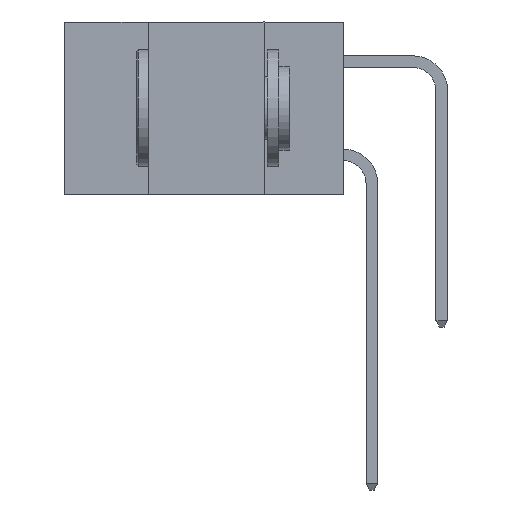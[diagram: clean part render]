
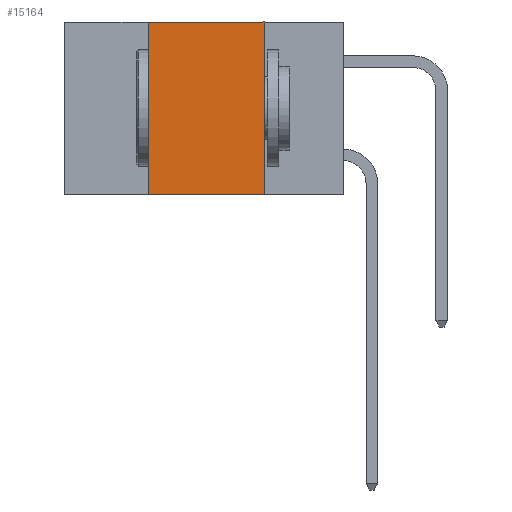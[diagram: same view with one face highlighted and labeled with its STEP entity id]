
A CAD part, left-side view. The second image highlights one B-rep face of the part: STEP entity #15164.
In plain terms, the highlighted planar face has unit normal (-1, 0, 0).
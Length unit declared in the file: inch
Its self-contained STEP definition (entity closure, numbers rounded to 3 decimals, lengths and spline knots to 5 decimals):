
#13 = DIRECTION ( 'NONE',  ( 0., 0., -1. ) ) ;
#141 = LINE ( 'NONE', #6042, #16493 ) ;
#431 = EDGE_CURVE ( 'NONE', #6835, #19722, #13069, .T. ) ;
#673 = ORIENTED_EDGE ( 'NONE', *, *, #8727, .F. ) ;
#1235 = CARTESIAN_POINT ( 'NONE',  ( 0., 0.42, -0.37 ) ) ;
#2145 = ORIENTED_EDGE ( 'NONE', *, *, #431, .T. ) ;
#2533 = EDGE_CURVE ( 'NONE', #6835, #9388, #14543, .T. ) ;
#3103 = PLANE ( 'NONE',  #10403 ) ;
#4089 = DIRECTION ( 'NONE',  ( 0., -1., 0. ) ) ;
#4337 = ORIENTED_EDGE ( 'NONE', *, *, #9751, .F. ) ;
#5850 = VERTEX_POINT ( 'NONE', #9584 ) ;
#5993 = VECTOR ( 'NONE', #4089, 39.37008 ) ;
#6042 = CARTESIAN_POINT ( 'NONE',  ( 0., 0.17, -0.37 ) ) ;
#6835 = VERTEX_POINT ( 'NONE', #10335 ) ;
#7136 = CARTESIAN_POINT ( 'NONE',  ( 0., 0.6, 0. ) ) ;
#7593 = DIRECTION ( 'NONE',  ( 0., 0., -1. ) ) ;
#7647 = CARTESIAN_POINT ( 'NONE',  ( 0., 0.6, -0.37 ) ) ;
#8727 = EDGE_CURVE ( 'NONE', #9388, #5850, #14105, .T. ) ;
#9280 = DIRECTION ( 'NONE',  ( 1., 0., 0. ) ) ;
#9388 = VERTEX_POINT ( 'NONE', #15934 ) ;
#9390 = ORIENTED_EDGE ( 'NONE', *, *, #2533, .F. ) ;
#9470 = CARTESIAN_POINT ( 'NONE',  ( 0., 0.17, -0.37 ) ) ;
#9584 = CARTESIAN_POINT ( 'NONE',  ( 0., 0.17, 0. ) ) ;
#9751 = EDGE_CURVE ( 'NONE', #5850, #19722, #141, .T. ) ;
#10335 = CARTESIAN_POINT ( 'NONE',  ( 0., 0.42, -0.37 ) ) ;
#10403 = AXIS2_PLACEMENT_3D ( 'NONE', #12274, #9280, #13 ) ;
#11241 = DIRECTION ( 'NONE',  ( 0., -1., 0. ) ) ;
#12026 = FACE_OUTER_BOUND ( 'NONE', #19530, .T. ) ;
#12274 = CARTESIAN_POINT ( 'NONE',  ( 0., 0.6, 0. ) ) ;
#12603 = VECTOR ( 'NONE', #11241, 39.37008 ) ;
#13069 = LINE ( 'NONE', #7647, #12603 ) ;
#14105 = LINE ( 'NONE', #7136, #5993 ) ;
#14543 = LINE ( 'NONE', #1235, #19088 ) ;
#15164 = ADVANCED_FACE ( 'NONE', ( #12026 ), #3103, .F. ) ;
#15934 = CARTESIAN_POINT ( 'NONE',  ( 0., 0.42, 0. ) ) ;
#16493 = VECTOR ( 'NONE', #7593, 39.37008 ) ;
#18035 = DIRECTION ( 'NONE',  ( 0., 0., 1. ) ) ;
#19088 = VECTOR ( 'NONE', #18035, 39.37008 ) ;
#19530 = EDGE_LOOP ( 'NONE', ( #4337, #673, #9390, #2145 ) ) ;
#19722 = VERTEX_POINT ( 'NONE', #9470 ) ;
